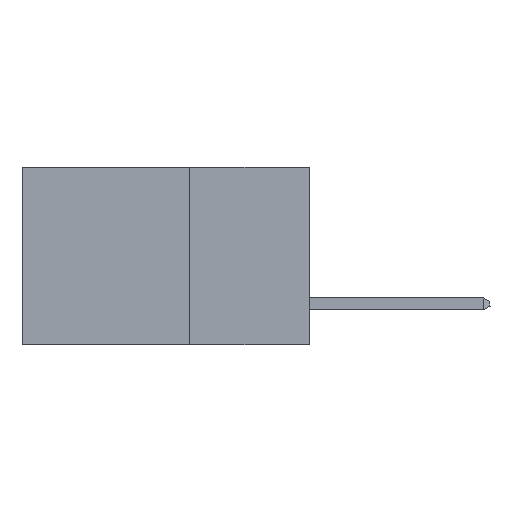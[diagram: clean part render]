
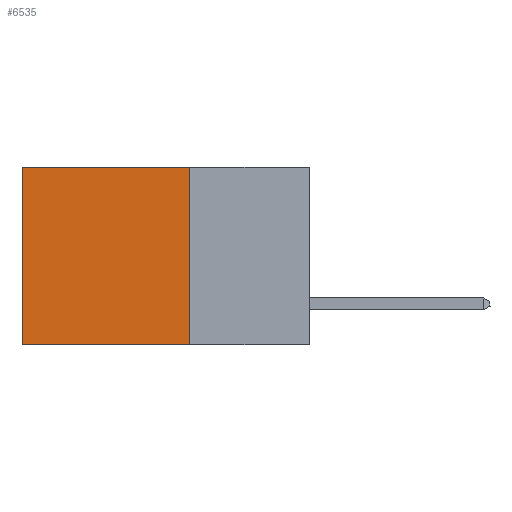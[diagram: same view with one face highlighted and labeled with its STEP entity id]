
A CAD part, left-side view. The second image highlights one B-rep face of the part: STEP entity #6535.
In plain terms, the highlighted planar face has unit normal (-1, 0, 0).
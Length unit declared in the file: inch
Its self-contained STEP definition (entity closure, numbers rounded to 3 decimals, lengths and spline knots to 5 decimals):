
#264 = FACE_OUTER_BOUND ( 'NONE', #11796, .T. ) ;
#523 = CARTESIAN_POINT ( 'NONE',  ( 0.2875, 0.25, -0.37 ) ) ;
#1946 = DIRECTION ( 'NONE',  ( 0., 0., -1. ) ) ;
#2157 = VERTEX_POINT ( 'NONE', #5601 ) ;
#2799 = DIRECTION ( 'NONE',  ( 0., 1., 0. ) ) ;
#3142 = EDGE_CURVE ( 'NONE', #2157, #9436, #24222, .T. ) ;
#3337 = ORIENTED_EDGE ( 'NONE', *, *, #20020, .T. ) ;
#4313 = PLANE ( 'NONE',  #11982 ) ;
#4993 = LINE ( 'NONE', #11168, #29272 ) ;
#5590 = EDGE_CURVE ( 'NONE', #23349, #9436, #18352, .T. ) ;
#5601 = CARTESIAN_POINT ( 'NONE',  ( 0.2875, 0.25, -0.37 ) ) ;
#5640 = CARTESIAN_POINT ( 'NONE',  ( 0.2875, 0.6, 0. ) ) ;
#6535 = ADVANCED_FACE ( 'NONE', ( #264 ), #4313, .F. ) ;
#8501 = DIRECTION ( 'NONE',  ( 0., 1., 0. ) ) ;
#8922 = VERTEX_POINT ( 'NONE', #20529 ) ;
#8936 = LINE ( 'NONE', #22090, #17297 ) ;
#9090 = DIRECTION ( 'NONE',  ( 0., 0., -1. ) ) ;
#9392 = ORIENTED_EDGE ( 'NONE', *, *, #3142, .F. ) ;
#9436 = VERTEX_POINT ( 'NONE', #24695 ) ;
#11168 = CARTESIAN_POINT ( 'NONE',  ( 0.2875, 0.25, 0. ) ) ;
#11517 = ORIENTED_EDGE ( 'NONE', *, *, #28750, .F. ) ;
#11796 = EDGE_LOOP ( 'NONE', ( #28286, #9392, #11517, #3337 ) ) ;
#11982 = AXIS2_PLACEMENT_3D ( 'NONE', #20727, #23377, #9090 ) ;
#12072 = VECTOR ( 'NONE', #22544, 39.37008 ) ;
#17297 = VECTOR ( 'NONE', #8501, 39.37008 ) ;
#18352 = LINE ( 'NONE', #27087, #12072 ) ;
#20020 = EDGE_CURVE ( 'NONE', #8922, #23349, #8936, .T. ) ;
#20529 = CARTESIAN_POINT ( 'NONE',  ( 0.2875, 0.25, 0. ) ) ;
#20727 = CARTESIAN_POINT ( 'NONE',  ( 0.2875, 0.25, 0. ) ) ;
#22090 = CARTESIAN_POINT ( 'NONE',  ( 0.2875, 0.25, 0. ) ) ;
#22544 = DIRECTION ( 'NONE',  ( 0., 0., -1. ) ) ;
#22793 = VECTOR ( 'NONE', #2799, 39.37008 ) ;
#23349 = VERTEX_POINT ( 'NONE', #5640 ) ;
#23377 = DIRECTION ( 'NONE',  ( 1., 0., 0. ) ) ;
#24222 = LINE ( 'NONE', #523, #22793 ) ;
#24695 = CARTESIAN_POINT ( 'NONE',  ( 0.2875, 0.6, -0.37 ) ) ;
#27087 = CARTESIAN_POINT ( 'NONE',  ( 0.2875, 0.6, 0. ) ) ;
#28286 = ORIENTED_EDGE ( 'NONE', *, *, #5590, .T. ) ;
#28750 = EDGE_CURVE ( 'NONE', #8922, #2157, #4993, .T. ) ;
#29272 = VECTOR ( 'NONE', #1946, 39.37008 ) ;
